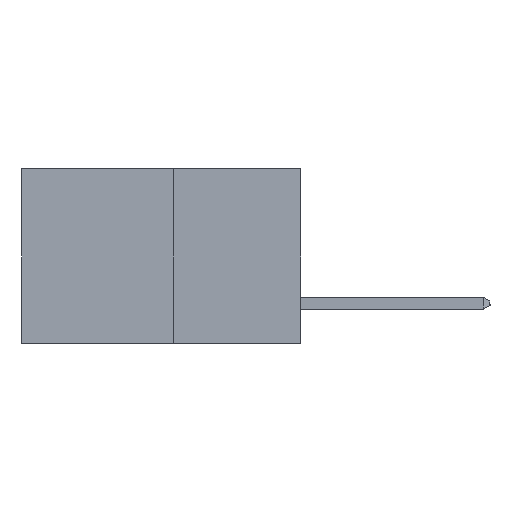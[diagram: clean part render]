
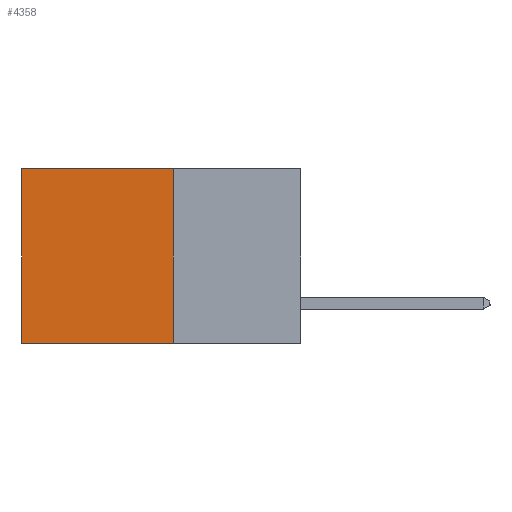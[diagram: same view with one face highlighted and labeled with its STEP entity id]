
A CAD part, left-side view. The second image highlights one B-rep face of the part: STEP entity #4358.
In plain terms, the highlighted planar face has unit normal (-1, 0, 0).
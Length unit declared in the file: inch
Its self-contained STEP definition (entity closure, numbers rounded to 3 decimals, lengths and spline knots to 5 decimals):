
#667 = DIRECTION ( 'NONE',  ( 0., 1., 0. ) ) ;
#896 = CARTESIAN_POINT ( 'NONE',  ( 0.277, 0.59, -0.37 ) ) ;
#1030 = CARTESIAN_POINT ( 'NONE',  ( 0.277, 0.27, 0. ) ) ;
#1184 = VERTEX_POINT ( 'NONE', #1030 ) ;
#1303 = ORIENTED_EDGE ( 'NONE', *, *, #4754, .F. ) ;
#1352 = ORIENTED_EDGE ( 'NONE', *, *, #12904, .T. ) ;
#1713 = EDGE_LOOP ( 'NONE', ( #4689, #10870, #1303, #1352 ) ) ;
#1936 = CARTESIAN_POINT ( 'NONE',  ( 0.277, 0.27, 0. ) ) ;
#2335 = LINE ( 'NONE', #13558, #5549 ) ;
#2418 = VERTEX_POINT ( 'NONE', #7641 ) ;
#2708 = LINE ( 'NONE', #11365, #14349 ) ;
#3120 = LINE ( 'NONE', #1936, #9120 ) ;
#4033 = LINE ( 'NONE', #8953, #6884 ) ;
#4164 = AXIS2_PLACEMENT_3D ( 'NONE', #4880, #6118, #14128 ) ;
#4358 = ADVANCED_FACE ( 'NONE', ( #12461 ), #11949, .F. ) ;
#4689 = ORIENTED_EDGE ( 'NONE', *, *, #14145, .T. ) ;
#4754 = EDGE_CURVE ( 'NONE', #1184, #2418, #4033, .T. ) ;
#4880 = CARTESIAN_POINT ( 'NONE',  ( 0.277, 0.27, -0.37 ) ) ;
#5529 = DIRECTION ( 'NONE',  ( 0., 1., 0. ) ) ;
#5549 = VECTOR ( 'NONE', #6709, 39.37008 ) ;
#6118 = DIRECTION ( 'NONE',  ( 1., 0., 0. ) ) ;
#6709 = DIRECTION ( 'NONE',  ( 0., 0., -1. ) ) ;
#6884 = VECTOR ( 'NONE', #7064, 39.37008 ) ;
#7064 = DIRECTION ( 'NONE',  ( 0., 0., -1. ) ) ;
#7641 = CARTESIAN_POINT ( 'NONE',  ( 0.277, 0.27, -0.37 ) ) ;
#8953 = CARTESIAN_POINT ( 'NONE',  ( 0.277, 0.27, -0.37 ) ) ;
#9120 = VECTOR ( 'NONE', #667, 39.37008 ) ;
#10586 = VERTEX_POINT ( 'NONE', #896 ) ;
#10870 = ORIENTED_EDGE ( 'NONE', *, *, #14163, .F. ) ;
#11365 = CARTESIAN_POINT ( 'NONE',  ( 0.277, 0.27, -0.37 ) ) ;
#11949 = PLANE ( 'NONE',  #4164 ) ;
#12461 = FACE_OUTER_BOUND ( 'NONE', #1713, .T. ) ;
#12904 = EDGE_CURVE ( 'NONE', #1184, #14687, #3120, .T. ) ;
#13558 = CARTESIAN_POINT ( 'NONE',  ( 0.277, 0.59, -0.37 ) ) ;
#14128 = DIRECTION ( 'NONE',  ( 0., 0., -1. ) ) ;
#14145 = EDGE_CURVE ( 'NONE', #14687, #10586, #2335, .T. ) ;
#14163 = EDGE_CURVE ( 'NONE', #2418, #10586, #2708, .T. ) ;
#14349 = VECTOR ( 'NONE', #5529, 39.37008 ) ;
#14448 = CARTESIAN_POINT ( 'NONE',  ( 0.277, 0.59, 0. ) ) ;
#14687 = VERTEX_POINT ( 'NONE', #14448 ) ;
